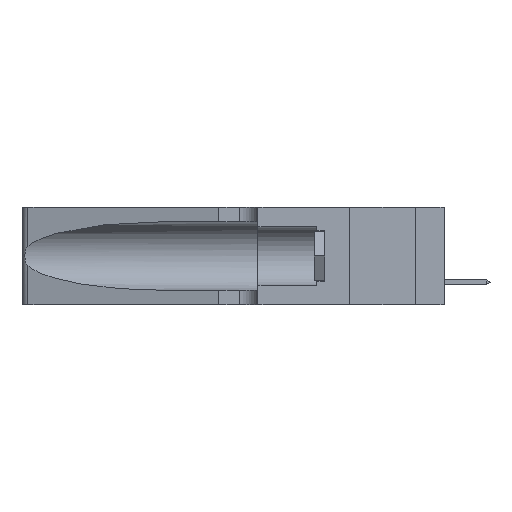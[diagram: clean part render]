
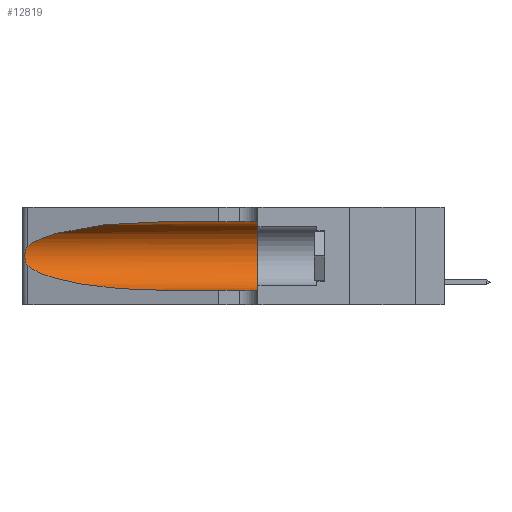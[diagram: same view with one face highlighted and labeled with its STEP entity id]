
A CAD part, left-side view. The second image highlights one B-rep face of the part: STEP entity #12819.
In plain terms, the highlighted cylindrical face has radius 3.308 mm (diameter 6.617 mm), a partial arc.
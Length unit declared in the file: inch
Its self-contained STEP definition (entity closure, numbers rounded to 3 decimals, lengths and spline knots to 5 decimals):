
#150 = VERTEX_POINT ( 'NONE', #36312 ) ;
#497 = CARTESIAN_POINT ( 'NONE',  ( 0.25487, 1.22718, 0.14631 ) ) ;
#580 = DIRECTION ( 'NONE',  ( 0., 1., 0. ) ) ;
#1370 = CARTESIAN_POINT ( 'NONE',  ( 0.25639, 1.23186, 0.15144 ) ) ;
#1899 = DIRECTION ( 'NONE',  ( 0., -1., 0. ) ) ;
#4308 = CARTESIAN_POINT ( 'NONE',  ( 0.1305, 0.35, 0.185 ) ) ;
#4443 = VECTOR ( 'NONE', #1899, 39.37008 ) ;
#4463 = ORIENTED_EDGE ( 'NONE', *, *, #39939, .T. ) ;
#4795 = CARTESIAN_POINT ( 'NONE',  ( 0.25856, 1.23593, 0.16098 ) ) ;
#5880 = ORIENTED_EDGE ( 'NONE', *, *, #16211, .T. ) ;
#6660 = EDGE_LOOP ( 'NONE', ( #5880, #18065, #14818, #4463, #17443, #31571 ) ) ;
#7156 = CYLINDRICAL_SURFACE ( 'NONE', #31589, 0.13025 ) ;
#8888 = CARTESIAN_POINT ( 'NONE',  ( 0.25555, 1.22993, 0.14849 ) ) ;
#10079 = CARTESIAN_POINT ( 'NONE',  ( 0.18966, 0.96281, 0.31525 ) ) ;
#10291 = DIRECTION ( 'NONE',  ( 0., -1., 0. ) ) ;
#12198 = CARTESIAN_POINT ( 'NONE',  ( 0.25789, 1.23486, 0.15765 ) ) ;
#12352 = CARTESIAN_POINT ( 'NONE',  ( 0.25787, 1.23484, 0.2124 ) ) ;
#12819 = ADVANCED_FACE ( 'NONE', ( #19561 ), #7156, .F. ) ;
#13901 = VERTEX_POINT ( 'NONE', #497 ) ;
#14571 = DIRECTION ( 'NONE',  ( 0., 0., 1. ) ) ;
#14818 = ORIENTED_EDGE ( 'NONE', *, *, #43500, .T. ) ;
#15347 = CARTESIAN_POINT ( 'NONE',  ( 0.25854, 1.2359, 0.20912 ) ) ;
#15463 =( BOUNDED_CURVE ( )  B_SPLINE_CURVE ( 3, ( #34409, #10079, #44171, #17126 ),
 .UNSPECIFIED., .F., .F. ) 
 B_SPLINE_CURVE_WITH_KNOTS ( ( 4, 4 ),
 ( 1.5708, 2.84003 ),
 .UNSPECIFIED. ) 
 CURVE ( )  GEOMETRIC_REPRESENTATION_ITEM ( )  RATIONAL_B_SPLINE_CURVE ( ( 1., 0.87, 0.87, 1. ) ) 
 REPRESENTATION_ITEM ( '' )  );
#15658 = CARTESIAN_POINT ( 'NONE',  ( 0.25639, 1.23184, 0.21858 ) ) ;
#16211 = EDGE_CURVE ( 'NONE', #28898, #150, #15463, .T. ) ;
#17126 = CARTESIAN_POINT ( 'NONE',  ( 0.25487, 1.22718, 0.22369 ) ) ;
#17443 = ORIENTED_EDGE ( 'NONE', *, *, #19543, .F. ) ;
#18065 = ORIENTED_EDGE ( 'NONE', *, *, #29383, .T. ) ;
#18150 = CARTESIAN_POINT ( 'NONE',  ( 0.2373, 1.15595, 0.08982 ) ) ;
#18782 = CARTESIAN_POINT ( 'NONE',  ( 0.26075, 1.23896, 0.19203 ) ) ;
#19438 = AXIS2_PLACEMENT_3D ( 'NONE', #4308, #580, #14571 ) ;
#19543 = EDGE_CURVE ( 'NONE', #40822, #32995, #44349, .T. ) ;
#19561 = FACE_OUTER_BOUND ( 'NONE', #6660, .T. ) ;
#20126 = B_SPLINE_CURVE_WITH_KNOTS ( 'NONE', 3,
 ( #29022, #22076, #15658, #12352, #15347, #39496, #18782, #29177, #35903, #4795, #12198, #1370, #8888, #25700 ),
 .UNSPECIFIED., .F., .F.,
 ( 4, 2, 2, 2, 2, 2, 4 ),
 ( 0., 0.00027, 0.00053, 0.00107, 0.0016, 0.00187, 0.00214 ),
 .UNSPECIFIED. ) ;
#21153 = CARTESIAN_POINT ( 'NONE',  ( 0.1305, 0.35, 0.05475 ) ) ;
#21701 = CARTESIAN_POINT ( 'NONE',  ( 0.1305, 0.72297, 0.05475 ) ) ;
#22076 = CARTESIAN_POINT ( 'NONE',  ( 0.25555, 1.22994, 0.2215 ) ) ;
#25700 = CARTESIAN_POINT ( 'NONE',  ( 0.25487, 1.22718, 0.14631 ) ) ;
#26996 = LINE ( 'NONE', #30885, #31330 ) ;
#28155 = LINE ( 'NONE', #29253, #4443 ) ;
#28549 = CARTESIAN_POINT ( 'NONE',  ( 0.1305, 0.72297, 0.05475 ) ) ;
#28898 = VERTEX_POINT ( 'NONE', #36257 ) ;
#29022 = CARTESIAN_POINT ( 'NONE',  ( 0.25487, 1.22718, 0.22369 ) ) ;
#29177 = CARTESIAN_POINT ( 'NONE',  ( 0.26075, 1.23896, 0.178 ) ) ;
#29253 = CARTESIAN_POINT ( 'NONE',  ( 0.1305, 1.61858, 0.05475 ) ) ;
#29383 = EDGE_CURVE ( 'NONE', #150, #13901, #20126, .T. ) ;
#30885 = CARTESIAN_POINT ( 'NONE',  ( 0.1305, 1.61858, 0.31525 ) ) ;
#30891 =( BOUNDED_CURVE ( )  B_SPLINE_CURVE ( 3, ( #38567, #18150, #42314, #28549 ),
 .UNSPECIFIED., .F., .T. ) 
 B_SPLINE_CURVE_WITH_KNOTS ( ( 4, 4 ),
 ( 3.44316, 4.71239 ),
 .UNSPECIFIED. ) 
 CURVE ( )  GEOMETRIC_REPRESENTATION_ITEM ( )  RATIONAL_B_SPLINE_CURVE ( ( 1., 0.87, 0.87, 1. ) ) 
 REPRESENTATION_ITEM ( '' )  );
#31330 = VECTOR ( 'NONE', #10291, 39.37008 ) ;
#31571 = ORIENTED_EDGE ( 'NONE', *, *, #41072, .F. ) ;
#31589 = AXIS2_PLACEMENT_3D ( 'NONE', #33338, #39912, #37068 ) ;
#32995 = VERTEX_POINT ( 'NONE', #21153 ) ;
#33338 = CARTESIAN_POINT ( 'NONE',  ( 0.1305, 1.61858, 0.185 ) ) ;
#34409 = CARTESIAN_POINT ( 'NONE',  ( 0.1305, 0.72297, 0.31525 ) ) ;
#35903 = CARTESIAN_POINT ( 'NONE',  ( 0.26017, 1.23833, 0.17102 ) ) ;
#36257 = CARTESIAN_POINT ( 'NONE',  ( 0.1305, 0.72297, 0.31525 ) ) ;
#36312 = CARTESIAN_POINT ( 'NONE',  ( 0.25487, 1.22718, 0.22369 ) ) ;
#37068 = DIRECTION ( 'NONE',  ( 0., 0., -1. ) ) ;
#38567 = CARTESIAN_POINT ( 'NONE',  ( 0.25487, 1.22718, 0.14631 ) ) ;
#39496 = CARTESIAN_POINT ( 'NONE',  ( 0.26018, 1.23835, 0.19895 ) ) ;
#39912 = DIRECTION ( 'NONE',  ( 0., -1., 0. ) ) ;
#39939 = EDGE_CURVE ( 'NONE', #44263, #32995, #28155, .T. ) ;
#40822 = VERTEX_POINT ( 'NONE', #40878 ) ;
#40878 = CARTESIAN_POINT ( 'NONE',  ( 0.1305, 0.35, 0.31525 ) ) ;
#41072 = EDGE_CURVE ( 'NONE', #28898, #40822, #26996, .T. ) ;
#42314 = CARTESIAN_POINT ( 'NONE',  ( 0.18966, 0.96281, 0.05475 ) ) ;
#43500 = EDGE_CURVE ( 'NONE', #13901, #44263, #30891, .T. ) ;
#44171 = CARTESIAN_POINT ( 'NONE',  ( 0.2373, 1.15595, 0.28018 ) ) ;
#44263 = VERTEX_POINT ( 'NONE', #21701 ) ;
#44349 = CIRCLE ( 'NONE', #19438, 0.13025 ) ;
